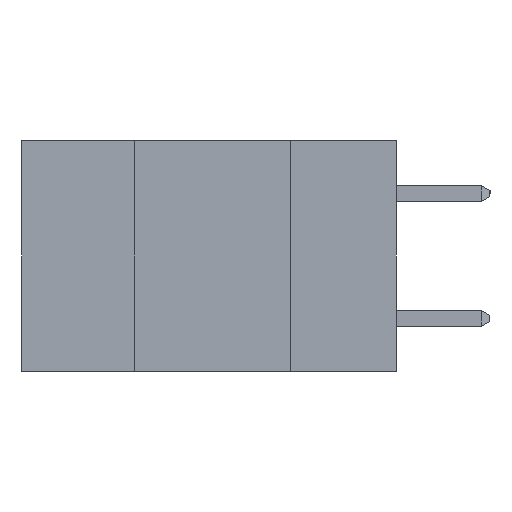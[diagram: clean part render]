
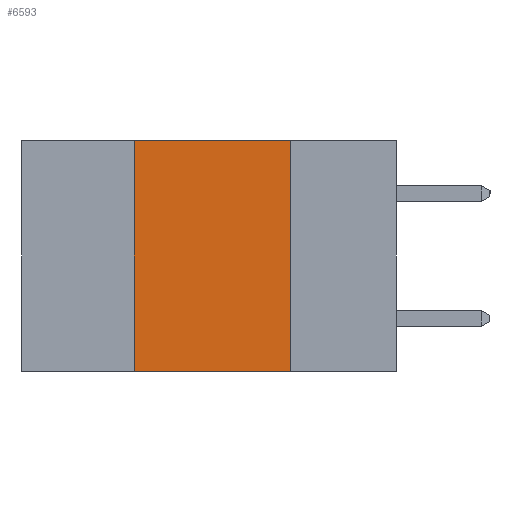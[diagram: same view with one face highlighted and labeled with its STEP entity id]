
A CAD part, left-side view. The second image highlights one B-rep face of the part: STEP entity #6593.
In plain terms, the highlighted planar face has unit normal (-1, 0, 0).
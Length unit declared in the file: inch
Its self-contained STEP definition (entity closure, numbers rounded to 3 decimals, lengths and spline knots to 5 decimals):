
#379 = DIRECTION ( 'NONE',  ( 0., 0., -1. ) ) ;
#854 = CARTESIAN_POINT ( 'NONE',  ( 0., 0.6, 0. ) ) ;
#1132 = CARTESIAN_POINT ( 'NONE',  ( 0., 0.42, -0.37 ) ) ;
#1425 = CARTESIAN_POINT ( 'NONE',  ( 0., 0.6, -0.37 ) ) ;
#1647 = VECTOR ( 'NONE', #14051, 39.37008 ) ;
#2273 = LINE ( 'NONE', #1425, #1647 ) ;
#2711 = EDGE_CURVE ( 'NONE', #4877, #10379, #8395, .T. ) ;
#3128 = LINE ( 'NONE', #9874, #3592 ) ;
#3220 = VERTEX_POINT ( 'NONE', #8661 ) ;
#3592 = VECTOR ( 'NONE', #13322, 39.37008 ) ;
#3858 = AXIS2_PLACEMENT_3D ( 'NONE', #854, #14455, #13536 ) ;
#4329 = VECTOR ( 'NONE', #379, 39.37008 ) ;
#4658 = ORIENTED_EDGE ( 'NONE', *, *, #4813, .T. ) ;
#4813 = EDGE_CURVE ( 'NONE', #12430, #10379, #2273, .T. ) ;
#4877 = VERTEX_POINT ( 'NONE', #12752 ) ;
#4893 = EDGE_CURVE ( 'NONE', #12430, #3220, #10606, .T. ) ;
#5071 = CARTESIAN_POINT ( 'NONE',  ( 0., 0.17, -0.37 ) ) ;
#6102 = EDGE_CURVE ( 'NONE', #3220, #4877, #3128, .T. ) ;
#6347 = EDGE_LOOP ( 'NONE', ( #7875, #10592, #11444, #4658 ) ) ;
#6593 = ADVANCED_FACE ( 'NONE', ( #14693 ), #8870, .F. ) ;
#7118 = DIRECTION ( 'NONE',  ( 0., 0., 1. ) ) ;
#7875 = ORIENTED_EDGE ( 'NONE', *, *, #2711, .F. ) ;
#8395 = LINE ( 'NONE', #5071, #4329 ) ;
#8661 = CARTESIAN_POINT ( 'NONE',  ( 0., 0.42, 0. ) ) ;
#8870 = PLANE ( 'NONE',  #3858 ) ;
#9874 = CARTESIAN_POINT ( 'NONE',  ( 0., 0.6, 0. ) ) ;
#10379 = VERTEX_POINT ( 'NONE', #11140 ) ;
#10592 = ORIENTED_EDGE ( 'NONE', *, *, #6102, .F. ) ;
#10606 = LINE ( 'NONE', #1132, #14771 ) ;
#11140 = CARTESIAN_POINT ( 'NONE',  ( 0., 0.17, -0.37 ) ) ;
#11444 = ORIENTED_EDGE ( 'NONE', *, *, #4893, .F. ) ;
#11730 = CARTESIAN_POINT ( 'NONE',  ( 0., 0.42, -0.37 ) ) ;
#12430 = VERTEX_POINT ( 'NONE', #11730 ) ;
#12752 = CARTESIAN_POINT ( 'NONE',  ( 0., 0.17, 0. ) ) ;
#13322 = DIRECTION ( 'NONE',  ( 0., -1., 0. ) ) ;
#13536 = DIRECTION ( 'NONE',  ( 0., 0., -1. ) ) ;
#14051 = DIRECTION ( 'NONE',  ( 0., -1., 0. ) ) ;
#14455 = DIRECTION ( 'NONE',  ( 1., 0., 0. ) ) ;
#14693 = FACE_OUTER_BOUND ( 'NONE', #6347, .T. ) ;
#14771 = VECTOR ( 'NONE', #7118, 39.37008 ) ;
